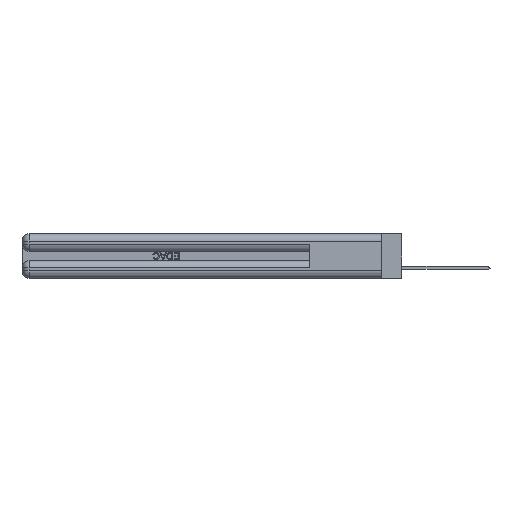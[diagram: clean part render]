
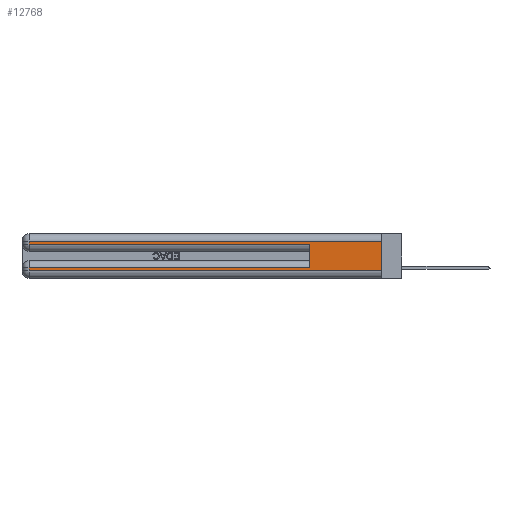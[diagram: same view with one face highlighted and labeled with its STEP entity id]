
A CAD part, left-side view. The second image highlights one B-rep face of the part: STEP entity #12768.
In plain terms, the highlighted planar face has unit normal (-1, 0, 0).
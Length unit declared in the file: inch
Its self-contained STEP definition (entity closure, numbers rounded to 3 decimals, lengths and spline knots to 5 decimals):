
#414 = LINE ( 'NONE', #31654, #20644 ) ;
#418 = VERTEX_POINT ( 'NONE', #7823 ) ;
#619 = ORIENTED_EDGE ( 'NONE', *, *, #33012, .T. ) ;
#666 = EDGE_CURVE ( 'NONE', #31257, #15303, #39562, .T. ) ;
#2484 = CARTESIAN_POINT ( 'NONE',  ( 0., 2.94, 0.37 ) ) ;
#3220 = DIRECTION ( 'NONE',  ( 1., 0., 0. ) ) ;
#3435 = ORIENTED_EDGE ( 'NONE', *, *, #9819, .F. ) ;
#4016 = EDGE_CURVE ( 'NONE', #27208, #42812, #17676, .T. ) ;
#4469 = CARTESIAN_POINT ( 'NONE',  ( 0., 0., 0.085 ) ) ;
#4534 = EDGE_CURVE ( 'NONE', #18685, #27208, #10718, .T. ) ;
#4902 = ORIENTED_EDGE ( 'NONE', *, *, #26886, .F. ) ;
#5033 = EDGE_LOOP ( 'NONE', ( #3435, #619, #23297, #29743, #4902, #13576, #23625, #28864 ) ) ;
#5197 = DIRECTION ( 'NONE',  ( 0., 0., -1. ) ) ;
#5555 = EDGE_CURVE ( 'NONE', #15303, #32173, #414, .T. ) ;
#7021 = VECTOR ( 'NONE', #16038, 39.37008 ) ;
#7425 = DIRECTION ( 'NONE',  ( 0., -1., 0. ) ) ;
#7823 = CARTESIAN_POINT ( 'NONE',  ( 0., 0., 0.31 ) ) ;
#9819 = EDGE_CURVE ( 'NONE', #418, #42812, #19954, .T. ) ;
#10718 = LINE ( 'NONE', #2484, #40459 ) ;
#12768 = ADVANCED_FACE ( 'NONE', ( #44412 ), #31179, .F. ) ;
#13173 = CARTESIAN_POINT ( 'NONE',  ( 0., 2.94, 0.37 ) ) ;
#13576 = ORIENTED_EDGE ( 'NONE', *, *, #36566, .T. ) ;
#13727 = VECTOR ( 'NONE', #30578, 39.37008 ) ;
#14177 = CARTESIAN_POINT ( 'NONE',  ( 0., 2.94, 0.06 ) ) ;
#15303 = VERTEX_POINT ( 'NONE', #19100 ) ;
#15359 = CARTESIAN_POINT ( 'NONE',  ( 0., 0., 0.06 ) ) ;
#16038 = DIRECTION ( 'NONE',  ( 0., -1., 0. ) ) ;
#17147 = DIRECTION ( 'NONE',  ( 0., 0., -1. ) ) ;
#17676 = LINE ( 'NONE', #15359, #7021 ) ;
#18685 = VERTEX_POINT ( 'NONE', #36031 ) ;
#19100 = CARTESIAN_POINT ( 'NONE',  ( 0., 2.94, 0.285 ) ) ;
#19434 = LINE ( 'NONE', #37623, #13727 ) ;
#19954 = LINE ( 'NONE', #28720, #30036 ) ;
#20486 = LINE ( 'NONE', #21725, #47804 ) ;
#20644 = VECTOR ( 'NONE', #7425, 39.37008 ) ;
#21182 = CARTESIAN_POINT ( 'NONE',  ( 0., 0., 0.06 ) ) ;
#21725 = CARTESIAN_POINT ( 'NONE',  ( 0., 0.6, 0.145 ) ) ;
#23297 = ORIENTED_EDGE ( 'NONE', *, *, #666, .T. ) ;
#23625 = ORIENTED_EDGE ( 'NONE', *, *, #4534, .T. ) ;
#26369 = AXIS2_PLACEMENT_3D ( 'NONE', #31700, #3220, #47657 ) ;
#26886 = EDGE_CURVE ( 'NONE', #42711, #32173, #20486, .T. ) ;
#27208 = VERTEX_POINT ( 'NONE', #14177 ) ;
#28720 = CARTESIAN_POINT ( 'NONE',  ( 0., 0., 0.37 ) ) ;
#28864 = ORIENTED_EDGE ( 'NONE', *, *, #4016, .T. ) ;
#29743 = ORIENTED_EDGE ( 'NONE', *, *, #5555, .T. ) ;
#30036 = VECTOR ( 'NONE', #17147, 39.37008 ) ;
#30578 = DIRECTION ( 'NONE',  ( 0., 1., 0. ) ) ;
#30806 = DIRECTION ( 'NONE',  ( 0., 0., -1. ) ) ;
#31179 = PLANE ( 'NONE',  #26369 ) ;
#31257 = VERTEX_POINT ( 'NONE', #40882 ) ;
#31654 = CARTESIAN_POINT ( 'NONE',  ( 0., 0., 0.285 ) ) ;
#31700 = CARTESIAN_POINT ( 'NONE',  ( 0., 0., 0.37 ) ) ;
#32173 = VERTEX_POINT ( 'NONE', #41229 ) ;
#32429 = VECTOR ( 'NONE', #36479, 39.37008 ) ;
#33012 = EDGE_CURVE ( 'NONE', #418, #31257, #19434, .T. ) ;
#36031 = CARTESIAN_POINT ( 'NONE',  ( 0., 2.94, 0.085 ) ) ;
#36479 = DIRECTION ( 'NONE',  ( 0., 1., 0. ) ) ;
#36566 = EDGE_CURVE ( 'NONE', #42711, #18685, #43222, .T. ) ;
#37623 = CARTESIAN_POINT ( 'NONE',  ( 0., 0., 0.31 ) ) ;
#39562 = LINE ( 'NONE', #13173, #46511 ) ;
#40459 = VECTOR ( 'NONE', #30806, 39.37008 ) ;
#40882 = CARTESIAN_POINT ( 'NONE',  ( 0., 2.94, 0.31 ) ) ;
#41229 = CARTESIAN_POINT ( 'NONE',  ( 0., 0.6, 0.285 ) ) ;
#42711 = VERTEX_POINT ( 'NONE', #50068 ) ;
#42812 = VERTEX_POINT ( 'NONE', #21182 ) ;
#43222 = LINE ( 'NONE', #4469, #32429 ) ;
#44412 = FACE_OUTER_BOUND ( 'NONE', #5033, .T. ) ;
#46511 = VECTOR ( 'NONE', #5197, 39.37008 ) ;
#47657 = DIRECTION ( 'NONE',  ( 0., 0., -1. ) ) ;
#47804 = VECTOR ( 'NONE', #49902, 39.37008 ) ;
#49902 = DIRECTION ( 'NONE',  ( 0., 0., 1. ) ) ;
#50068 = CARTESIAN_POINT ( 'NONE',  ( 0., 0.6, 0.085 ) ) ;
